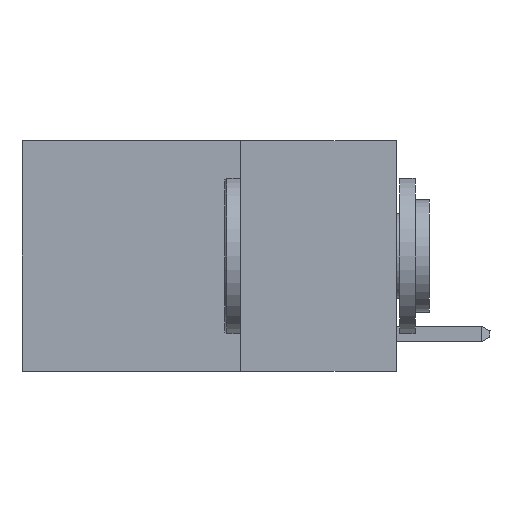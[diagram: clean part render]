
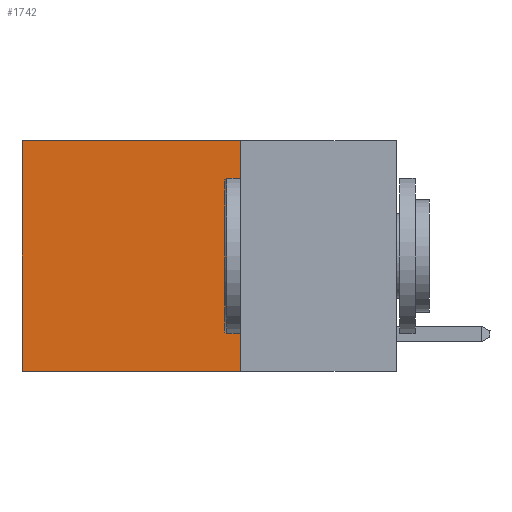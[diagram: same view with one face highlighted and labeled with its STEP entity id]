
A CAD part, left-side view. The second image highlights one B-rep face of the part: STEP entity #1742.
In plain terms, the highlighted planar face has unit normal (-1, 0, 0).
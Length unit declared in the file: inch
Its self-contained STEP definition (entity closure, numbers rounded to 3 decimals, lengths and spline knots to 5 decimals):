
#321 = EDGE_CURVE ( 'NONE', #6092, #4303, #22891, .T. ) ;
#550 = CARTESIAN_POINT ( 'NONE',  ( 0.2625, 0.25, -0.37 ) ) ;
#1174 = LINE ( 'NONE', #13024, #15580 ) ;
#1742 = ADVANCED_FACE ( 'NONE', ( #7735 ), #23917, .F. ) ;
#3850 = EDGE_CURVE ( 'NONE', #22569, #6790, #17961, .T. ) ;
#4178 = DIRECTION ( 'NONE',  ( 0., 0., -1. ) ) ;
#4303 = VERTEX_POINT ( 'NONE', #6761 ) ;
#4736 = VECTOR ( 'NONE', #4178, 39.37008 ) ;
#6092 = VERTEX_POINT ( 'NONE', #15083 ) ;
#6761 = CARTESIAN_POINT ( 'NONE',  ( 0.2625, 0.25, -0.37 ) ) ;
#6790 = VERTEX_POINT ( 'NONE', #22960 ) ;
#7735 = FACE_OUTER_BOUND ( 'NONE', #17419, .T. ) ;
#7936 = DIRECTION ( 'NONE',  ( 0., 1., 0. ) ) ;
#9572 = EDGE_CURVE ( 'NONE', #6092, #22569, #1174, .T. ) ;
#10869 = VECTOR ( 'NONE', #21200, 39.37008 ) ;
#11233 = ORIENTED_EDGE ( 'NONE', *, *, #3850, .T. ) ;
#11713 = EDGE_CURVE ( 'NONE', #4303, #6790, #27518, .T. ) ;
#12634 = ORIENTED_EDGE ( 'NONE', *, *, #321, .F. ) ;
#13024 = CARTESIAN_POINT ( 'NONE',  ( 0.2625, 0.25, 0. ) ) ;
#14841 = AXIS2_PLACEMENT_3D ( 'NONE', #23076, #24067, #20820 ) ;
#15083 = CARTESIAN_POINT ( 'NONE',  ( 0.2625, 0.25, 0. ) ) ;
#15580 = VECTOR ( 'NONE', #7936, 39.37008 ) ;
#15850 = DIRECTION ( 'NONE',  ( 0., 0., -1. ) ) ;
#17419 = EDGE_LOOP ( 'NONE', ( #11233, #21682, #12634, #24221 ) ) ;
#17961 = LINE ( 'NONE', #24714, #4736 ) ;
#18074 = CARTESIAN_POINT ( 'NONE',  ( 0.2625, 0.25, 0. ) ) ;
#20820 = DIRECTION ( 'NONE',  ( 0., 0., -1. ) ) ;
#21200 = DIRECTION ( 'NONE',  ( 0., 1., 0. ) ) ;
#21682 = ORIENTED_EDGE ( 'NONE', *, *, #11713, .F. ) ;
#22569 = VERTEX_POINT ( 'NONE', #28456 ) ;
#22891 = LINE ( 'NONE', #18074, #27988 ) ;
#22960 = CARTESIAN_POINT ( 'NONE',  ( 0.2625, 0.6, -0.37 ) ) ;
#23076 = CARTESIAN_POINT ( 'NONE',  ( 0.2625, 0.25, 0. ) ) ;
#23917 = PLANE ( 'NONE',  #14841 ) ;
#24067 = DIRECTION ( 'NONE',  ( 1., 0., 0. ) ) ;
#24221 = ORIENTED_EDGE ( 'NONE', *, *, #9572, .T. ) ;
#24714 = CARTESIAN_POINT ( 'NONE',  ( 0.2625, 0.6, 0. ) ) ;
#27518 = LINE ( 'NONE', #550, #10869 ) ;
#27988 = VECTOR ( 'NONE', #15850, 39.37008 ) ;
#28456 = CARTESIAN_POINT ( 'NONE',  ( 0.2625, 0.6, 0. ) ) ;
